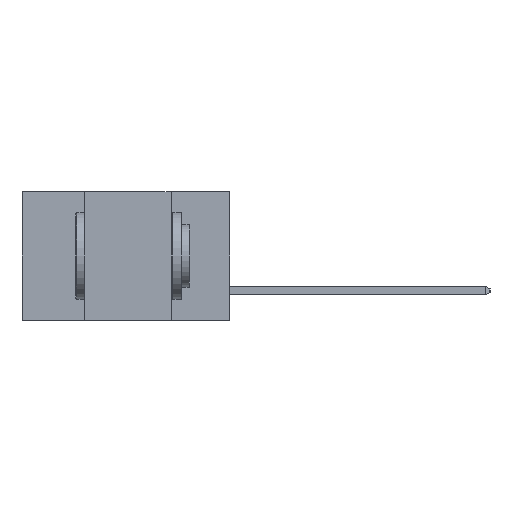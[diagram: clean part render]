
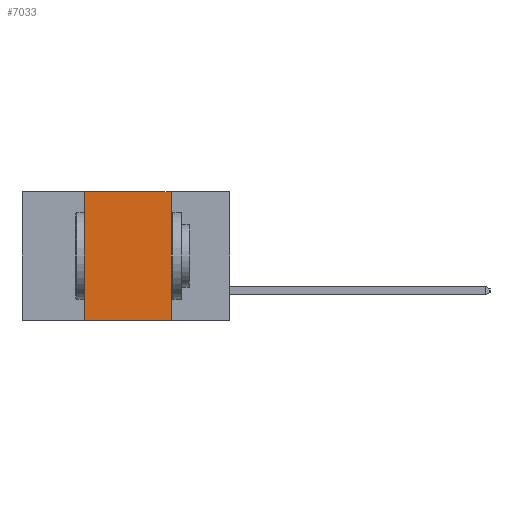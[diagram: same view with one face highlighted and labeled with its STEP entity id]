
A CAD part, left-side view. The second image highlights one B-rep face of the part: STEP entity #7033.
In plain terms, the highlighted planar face has unit normal (-1, 0, 0).
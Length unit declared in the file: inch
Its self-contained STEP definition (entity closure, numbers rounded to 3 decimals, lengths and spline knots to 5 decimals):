
#208 = CARTESIAN_POINT ( 'NONE',  ( 0., 0.17, 0. ) ) ;
#614 = VECTOR ( 'NONE', #12521, 39.37008 ) ;
#843 = DIRECTION ( 'NONE',  ( 0., 0., -1. ) ) ;
#1237 = DIRECTION ( 'NONE',  ( 1., 0., 0. ) ) ;
#1379 = CARTESIAN_POINT ( 'NONE',  ( 0., 0.6, -0.37 ) ) ;
#2166 = VECTOR ( 'NONE', #8848, 39.37008 ) ;
#2567 = LINE ( 'NONE', #5988, #5391 ) ;
#2644 = CARTESIAN_POINT ( 'NONE',  ( 0., 0.17, 0. ) ) ;
#3324 = VERTEX_POINT ( 'NONE', #9248 ) ;
#3463 = EDGE_CURVE ( 'NONE', #6421, #9815, #6728, .T. ) ;
#3733 = ORIENTED_EDGE ( 'NONE', *, *, #3463, .F. ) ;
#4103 = VECTOR ( 'NONE', #11540, 39.37008 ) ;
#4157 = CARTESIAN_POINT ( 'NONE',  ( 0., 0.17, -0.37 ) ) ;
#4404 = ORIENTED_EDGE ( 'NONE', *, *, #11664, .F. ) ;
#4709 = VERTEX_POINT ( 'NONE', #9249 ) ;
#5251 = ORIENTED_EDGE ( 'NONE', *, *, #13119, .F. ) ;
#5391 = VECTOR ( 'NONE', #12344, 39.37008 ) ;
#5965 = PLANE ( 'NONE',  #12886 ) ;
#5988 = CARTESIAN_POINT ( 'NONE',  ( 0., 0.42, 0. ) ) ;
#6421 = VERTEX_POINT ( 'NONE', #2644 ) ;
#6728 = LINE ( 'NONE', #208, #4103 ) ;
#6836 = CARTESIAN_POINT ( 'NONE',  ( 0., 0.6, 0. ) ) ;
#7033 = ADVANCED_FACE ( 'NONE', ( #8351 ), #5965, .F. ) ;
#8351 = FACE_OUTER_BOUND ( 'NONE', #13257, .T. ) ;
#8848 = DIRECTION ( 'NONE',  ( 0., -1., 0. ) ) ;
#9060 = LINE ( 'NONE', #11488, #614 ) ;
#9248 = CARTESIAN_POINT ( 'NONE',  ( 0., 0.42, -0.37 ) ) ;
#9249 = CARTESIAN_POINT ( 'NONE',  ( 0., 0.42, 0. ) ) ;
#9501 = EDGE_CURVE ( 'NONE', #3324, #9815, #13374, .T. ) ;
#9815 = VERTEX_POINT ( 'NONE', #4157 ) ;
#11488 = CARTESIAN_POINT ( 'NONE',  ( 0., 0.6, 0. ) ) ;
#11540 = DIRECTION ( 'NONE',  ( 0., 0., -1. ) ) ;
#11664 = EDGE_CURVE ( 'NONE', #3324, #4709, #2567, .T. ) ;
#11731 = ORIENTED_EDGE ( 'NONE', *, *, #9501, .T. ) ;
#12344 = DIRECTION ( 'NONE',  ( 0., 0., 1. ) ) ;
#12521 = DIRECTION ( 'NONE',  ( 0., -1., 0. ) ) ;
#12886 = AXIS2_PLACEMENT_3D ( 'NONE', #6836, #1237, #843 ) ;
#13119 = EDGE_CURVE ( 'NONE', #4709, #6421, #9060, .T. ) ;
#13257 = EDGE_LOOP ( 'NONE', ( #3733, #5251, #4404, #11731 ) ) ;
#13374 = LINE ( 'NONE', #1379, #2166 ) ;
